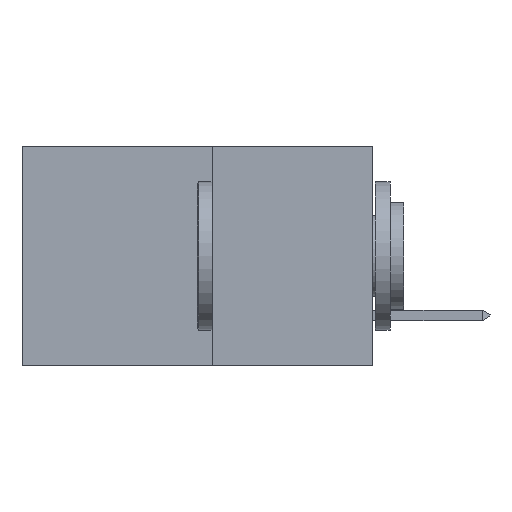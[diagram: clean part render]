
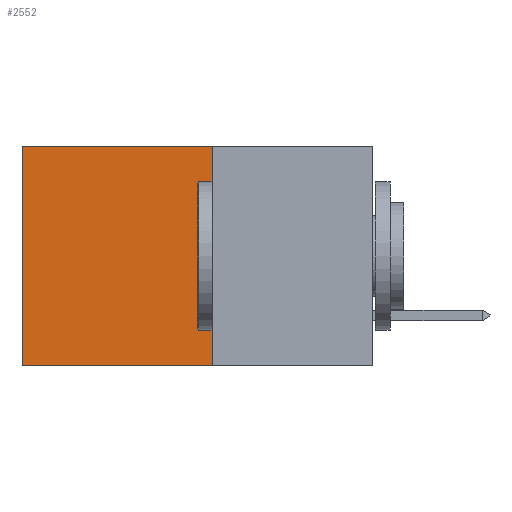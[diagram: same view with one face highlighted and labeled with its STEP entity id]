
A CAD part, left-side view. The second image highlights one B-rep face of the part: STEP entity #2552.
In plain terms, the highlighted planar face has unit normal (-1, 0, 0).
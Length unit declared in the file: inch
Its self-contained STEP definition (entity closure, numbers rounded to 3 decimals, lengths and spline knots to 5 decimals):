
#103 = EDGE_CURVE ( 'NONE', #10214, #6824, #10720, .T. ) ;
#307 = CARTESIAN_POINT ( 'NONE',  ( 0.277, 0.27, -0.37 ) ) ;
#719 = LINE ( 'NONE', #1758, #6166 ) ;
#771 = CARTESIAN_POINT ( 'NONE',  ( 0.277, 0.27, -0.37 ) ) ;
#1060 = EDGE_CURVE ( 'NONE', #2484, #10214, #719, .T. ) ;
#1682 = VECTOR ( 'NONE', #6878, 39.37008 ) ;
#1758 = CARTESIAN_POINT ( 'NONE',  ( 0.277, 0.27, 0. ) ) ;
#1800 = DIRECTION ( 'NONE',  ( 0., 1., 0. ) ) ;
#1848 = DIRECTION ( 'NONE',  ( 0., 0., -1. ) ) ;
#2484 = VERTEX_POINT ( 'NONE', #11071 ) ;
#2540 = CARTESIAN_POINT ( 'NONE',  ( 0.277, 0.59, -0.37 ) ) ;
#2552 = ADVANCED_FACE ( 'NONE', ( #11583 ), #3046, .F. ) ;
#3038 = CARTESIAN_POINT ( 'NONE',  ( 0.277, 0.27, -0.37 ) ) ;
#3046 = PLANE ( 'NONE',  #8453 ) ;
#3654 = DIRECTION ( 'NONE',  ( 0., 0., -1. ) ) ;
#4193 = CARTESIAN_POINT ( 'NONE',  ( 0.277, 0.27, -0.37 ) ) ;
#4408 = LINE ( 'NONE', #771, #1682 ) ;
#4430 = CARTESIAN_POINT ( 'NONE',  ( 0.277, 0.59, -0.37 ) ) ;
#5134 = ORIENTED_EDGE ( 'NONE', *, *, #1060, .T. ) ;
#5603 = VECTOR ( 'NONE', #1848, 39.37008 ) ;
#6166 = VECTOR ( 'NONE', #1800, 39.37008 ) ;
#6824 = VERTEX_POINT ( 'NONE', #4430 ) ;
#6878 = DIRECTION ( 'NONE',  ( 0., 0., -1. ) ) ;
#7177 = DIRECTION ( 'NONE',  ( 0., 1., 0. ) ) ;
#7429 = LINE ( 'NONE', #4193, #11904 ) ;
#7734 = ORIENTED_EDGE ( 'NONE', *, *, #7930, .F. ) ;
#7824 = VERTEX_POINT ( 'NONE', #3038 ) ;
#7930 = EDGE_CURVE ( 'NONE', #7824, #6824, #7429, .T. ) ;
#8453 = AXIS2_PLACEMENT_3D ( 'NONE', #307, #11939, #3654 ) ;
#8643 = ORIENTED_EDGE ( 'NONE', *, *, #103, .T. ) ;
#8944 = ORIENTED_EDGE ( 'NONE', *, *, #12009, .F. ) ;
#10214 = VERTEX_POINT ( 'NONE', #10741 ) ;
#10720 = LINE ( 'NONE', #2540, #5603 ) ;
#10741 = CARTESIAN_POINT ( 'NONE',  ( 0.277, 0.59, 0. ) ) ;
#11071 = CARTESIAN_POINT ( 'NONE',  ( 0.277, 0.27, 0. ) ) ;
#11583 = FACE_OUTER_BOUND ( 'NONE', #11592, .T. ) ;
#11592 = EDGE_LOOP ( 'NONE', ( #8643, #7734, #8944, #5134 ) ) ;
#11904 = VECTOR ( 'NONE', #7177, 39.37008 ) ;
#11939 = DIRECTION ( 'NONE',  ( 1., 0., 0. ) ) ;
#12009 = EDGE_CURVE ( 'NONE', #2484, #7824, #4408, .T. ) ;
